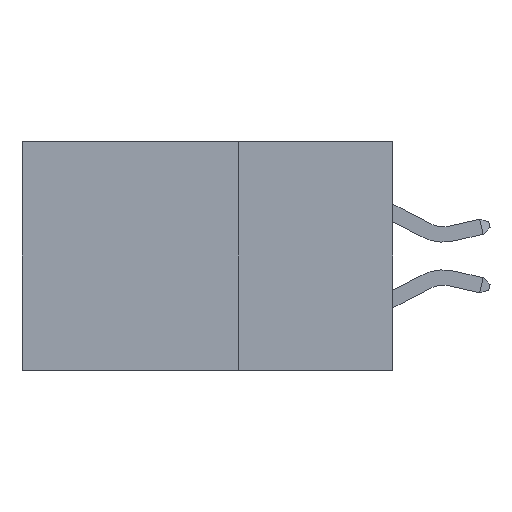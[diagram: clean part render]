
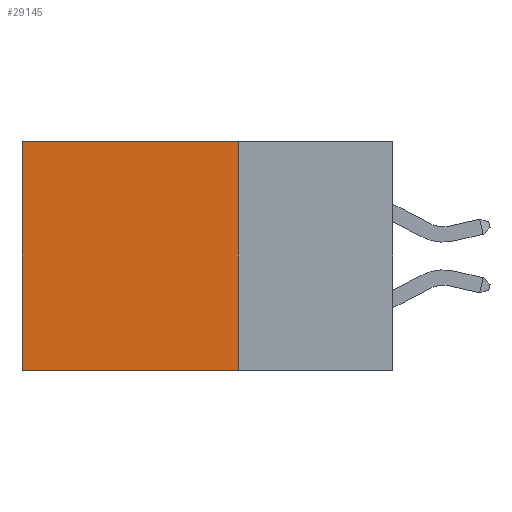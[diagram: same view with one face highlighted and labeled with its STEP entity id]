
A CAD part, left-side view. The second image highlights one B-rep face of the part: STEP entity #29145.
In plain terms, the highlighted planar face has unit normal (-1, 0, 0).
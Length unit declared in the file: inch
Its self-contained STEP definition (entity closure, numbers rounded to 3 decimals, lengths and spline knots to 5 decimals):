
#2037 = PLANE ( 'NONE',  #3361 ) ;
#2138 = ORIENTED_EDGE ( 'NONE', *, *, #7225, .F. ) ;
#2154 = LINE ( 'NONE', #34555, #8839 ) ;
#3361 = AXIS2_PLACEMENT_3D ( 'NONE', #34946, #21480, #4983 ) ;
#3590 = CARTESIAN_POINT ( 'NONE',  ( 0.2875, 0.6, 0. ) ) ;
#3599 = ORIENTED_EDGE ( 'NONE', *, *, #30691, .T. ) ;
#3937 = ORIENTED_EDGE ( 'NONE', *, *, #25507, .T. ) ;
#4983 = DIRECTION ( 'NONE',  ( 0., 0., -1. ) ) ;
#6256 = CARTESIAN_POINT ( 'NONE',  ( 0.2875, 0.25, 0. ) ) ;
#7225 = EDGE_CURVE ( 'NONE', #32648, #15821, #31428, .T. ) ;
#8081 = CARTESIAN_POINT ( 'NONE',  ( 0.2875, 0.6, 0. ) ) ;
#8839 = VECTOR ( 'NONE', #15603, 39.37008 ) ;
#9680 = LINE ( 'NONE', #3590, #29731 ) ;
#14030 = VERTEX_POINT ( 'NONE', #8081 ) ;
#15603 = DIRECTION ( 'NONE',  ( 0., 1., 0. ) ) ;
#15821 = VERTEX_POINT ( 'NONE', #22657 ) ;
#16610 = CARTESIAN_POINT ( 'NONE',  ( 0.2875, 0.25, 0. ) ) ;
#17486 = DIRECTION ( 'NONE',  ( 0., 0., -1. ) ) ;
#18740 = VECTOR ( 'NONE', #21956, 39.37008 ) ;
#20240 = LINE ( 'NONE', #24147, #33760 ) ;
#21480 = DIRECTION ( 'NONE',  ( 1., 0., 0. ) ) ;
#21956 = DIRECTION ( 'NONE',  ( 0., 0., -1. ) ) ;
#22657 = CARTESIAN_POINT ( 'NONE',  ( 0.2875, 0.25, -0.37 ) ) ;
#22935 = VERTEX_POINT ( 'NONE', #31166 ) ;
#24147 = CARTESIAN_POINT ( 'NONE',  ( 0.2875, 0.25, 0. ) ) ;
#25507 = EDGE_CURVE ( 'NONE', #32648, #14030, #20240, .T. ) ;
#26643 = ORIENTED_EDGE ( 'NONE', *, *, #30241, .F. ) ;
#27864 = FACE_OUTER_BOUND ( 'NONE', #35255, .T. ) ;
#29145 = ADVANCED_FACE ( 'NONE', ( #27864 ), #2037, .F. ) ;
#29731 = VECTOR ( 'NONE', #17486, 39.37008 ) ;
#30241 = EDGE_CURVE ( 'NONE', #15821, #22935, #2154, .T. ) ;
#30691 = EDGE_CURVE ( 'NONE', #14030, #22935, #9680, .T. ) ;
#31166 = CARTESIAN_POINT ( 'NONE',  ( 0.2875, 0.6, -0.37 ) ) ;
#31428 = LINE ( 'NONE', #16610, #18740 ) ;
#32335 = DIRECTION ( 'NONE',  ( 0., 1., 0. ) ) ;
#32648 = VERTEX_POINT ( 'NONE', #6256 ) ;
#33760 = VECTOR ( 'NONE', #32335, 39.37008 ) ;
#34555 = CARTESIAN_POINT ( 'NONE',  ( 0.2875, 0.25, -0.37 ) ) ;
#34946 = CARTESIAN_POINT ( 'NONE',  ( 0.2875, 0.25, 0. ) ) ;
#35255 = EDGE_LOOP ( 'NONE', ( #3599, #26643, #2138, #3937 ) ) ;
